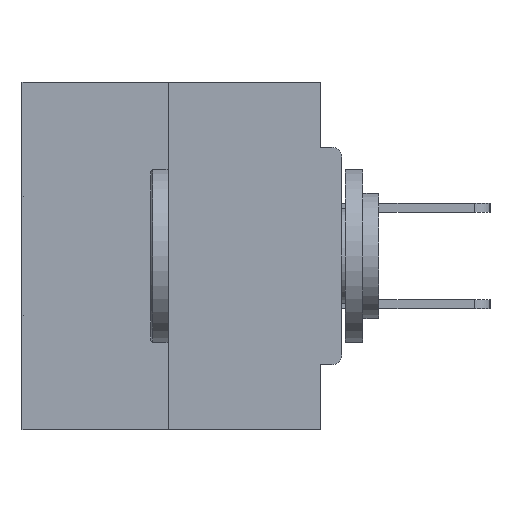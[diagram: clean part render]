
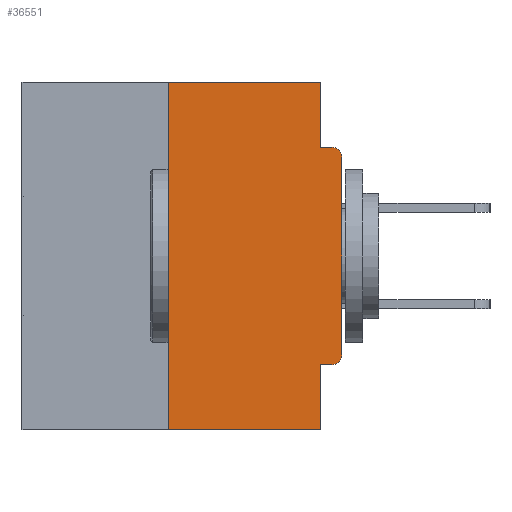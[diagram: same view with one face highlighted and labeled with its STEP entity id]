
A CAD part, left-side view. The second image highlights one B-rep face of the part: STEP entity #36551.
In plain terms, the highlighted planar face has unit normal (-1, 0, 0).
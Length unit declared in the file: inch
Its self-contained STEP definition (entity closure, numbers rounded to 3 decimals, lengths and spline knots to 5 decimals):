
#338 = DIRECTION ( 'NONE',  ( 0., -1., 0. ) ) ;
#385 = VECTOR ( 'NONE', #25717, 39.37008 ) ;
#518 = CARTESIAN_POINT ( 'NONE',  ( 0., 0.46, 0. ) ) ;
#1648 = DIRECTION ( 'NONE',  ( 0., 0., 1. ) ) ;
#1758 = CARTESIAN_POINT ( 'NONE',  ( 0., 0., 0. ) ) ;
#1766 = AXIS2_PLACEMENT_3D ( 'NONE', #30039, #36216, #30303 ) ;
#2018 = LINE ( 'NONE', #14596, #20647 ) ;
#2046 = CARTESIAN_POINT ( 'NONE',  ( 0., 0.25, -0.5 ) ) ;
#3592 = EDGE_CURVE ( 'NONE', #36708, #32702, #34409, .T. ) ;
#4123 = ORIENTED_EDGE ( 'NONE', *, *, #37410, .F. ) ;
#4656 = VECTOR ( 'NONE', #34241, 39.37008 ) ;
#4747 = CIRCLE ( 'NONE', #18517, 0.015 ) ;
#5923 = VERTEX_POINT ( 'NONE', #27540 ) ;
#6264 = CARTESIAN_POINT ( 'NONE',  ( 0., 0., -0.0935 ) ) ;
#6756 = VECTOR ( 'NONE', #338, 39.37008 ) ;
#6948 = ORIENTED_EDGE ( 'NONE', *, *, #17255, .F. ) ;
#7459 = DIRECTION ( 'NONE',  ( 1., 0., 0. ) ) ;
#8362 = EDGE_CURVE ( 'NONE', #36708, #20946, #20448, .T. ) ;
#8731 = CARTESIAN_POINT ( 'NONE',  ( 0., 0., -0.4065 ) ) ;
#9077 = LINE ( 'NONE', #6264, #6756 ) ;
#9250 = VERTEX_POINT ( 'NONE', #34932 ) ;
#9706 = ORIENTED_EDGE ( 'NONE', *, *, #15692, .T. ) ;
#9773 = VERTEX_POINT ( 'NONE', #11097 ) ;
#10700 = CARTESIAN_POINT ( 'NONE',  ( 0., 0.46, 0. ) ) ;
#11097 = CARTESIAN_POINT ( 'NONE',  ( 0., 0.015, -0.0935 ) ) ;
#11478 = LINE ( 'NONE', #518, #29188 ) ;
#11847 = CARTESIAN_POINT ( 'NONE',  ( 0., 0.031, -0.5 ) ) ;
#11968 = VECTOR ( 'NONE', #1648, 39.37008 ) ;
#11971 = CARTESIAN_POINT ( 'NONE',  ( 0., 0.015, -0.3915 ) ) ;
#12095 = DIRECTION ( 'NONE',  ( -1., 0., 0. ) ) ;
#14596 = CARTESIAN_POINT ( 'NONE',  ( 0., 0.031, 0. ) ) ;
#15692 = EDGE_CURVE ( 'NONE', #20719, #9773, #34105, .T. ) ;
#16983 = CARTESIAN_POINT ( 'NONE',  ( 0., 0.25, 0. ) ) ;
#17255 = EDGE_CURVE ( 'NONE', #5923, #20946, #37753, .T. ) ;
#17646 = CARTESIAN_POINT ( 'NONE',  ( 0., 0.015, -0.4065 ) ) ;
#18517 = AXIS2_PLACEMENT_3D ( 'NONE', #11971, #12095, #35986 ) ;
#19085 = ORIENTED_EDGE ( 'NONE', *, *, #19563, .F. ) ;
#19365 = PLANE ( 'NONE',  #24230 ) ;
#19563 = EDGE_CURVE ( 'NONE', #9250, #9773, #9077, .T. ) ;
#19780 = ORIENTED_EDGE ( 'NONE', *, *, #8362, .T. ) ;
#19796 = EDGE_CURVE ( 'NONE', #27564, #20719, #30009, .T. ) ;
#20267 = EDGE_LOOP ( 'NONE', ( #32837, #20473, #19780, #6948, #32783, #22545, #23385, #9706, #19085, #4123 ) ) ;
#20448 = LINE ( 'NONE', #31205, #4656 ) ;
#20473 = ORIENTED_EDGE ( 'NONE', *, *, #3592, .F. ) ;
#20647 = VECTOR ( 'NONE', #20677, 39.37008 ) ;
#20677 = DIRECTION ( 'NONE',  ( 0., 0., -1. ) ) ;
#20719 = VERTEX_POINT ( 'NONE', #34102 ) ;
#20946 = VERTEX_POINT ( 'NONE', #11847 ) ;
#20996 = EDGE_CURVE ( 'NONE', #27546, #5923, #31679, .T. ) ;
#21821 = VECTOR ( 'NONE', #32972, 39.37008 ) ;
#22545 = ORIENTED_EDGE ( 'NONE', *, *, #34361, .T. ) ;
#23385 = ORIENTED_EDGE ( 'NONE', *, *, #19796, .T. ) ;
#24230 = AXIS2_PLACEMENT_3D ( 'NONE', #10700, #7459, #31681 ) ;
#24546 = VERTEX_POINT ( 'NONE', #31802 ) ;
#25610 = DIRECTION ( 'NONE',  ( 0., 0., 1. ) ) ;
#25717 = DIRECTION ( 'NONE',  ( 0., 0., -1. ) ) ;
#25827 = FACE_OUTER_BOUND ( 'NONE', #20267, .T. ) ;
#26524 = CARTESIAN_POINT ( 'NONE',  ( 0., 0., -0.3915 ) ) ;
#27540 = CARTESIAN_POINT ( 'NONE',  ( 0., 0.031, -0.4065 ) ) ;
#27546 = VERTEX_POINT ( 'NONE', #17646 ) ;
#27564 = VERTEX_POINT ( 'NONE', #26524 ) ;
#28493 = CARTESIAN_POINT ( 'NONE',  ( 0., 0.031, -0.5 ) ) ;
#29188 = VECTOR ( 'NONE', #33545, 39.37008 ) ;
#30009 = LINE ( 'NONE', #1758, #32344 ) ;
#30039 = CARTESIAN_POINT ( 'NONE',  ( 0., 0.015, -0.1085 ) ) ;
#30303 = DIRECTION ( 'NONE',  ( 0., 0., -1. ) ) ;
#31205 = CARTESIAN_POINT ( 'NONE',  ( 0., 0.46, -0.5 ) ) ;
#31679 = LINE ( 'NONE', #8731, #21821 ) ;
#31681 = DIRECTION ( 'NONE',  ( 0., 0., -1. ) ) ;
#31802 = CARTESIAN_POINT ( 'NONE',  ( 0., 0.031, 0. ) ) ;
#32344 = VECTOR ( 'NONE', #25610, 39.37008 ) ;
#32702 = VERTEX_POINT ( 'NONE', #16983 ) ;
#32783 = ORIENTED_EDGE ( 'NONE', *, *, #20996, .F. ) ;
#32837 = ORIENTED_EDGE ( 'NONE', *, *, #35759, .F. ) ;
#32972 = DIRECTION ( 'NONE',  ( 0., 1., 0. ) ) ;
#33545 = DIRECTION ( 'NONE',  ( 0., -1., 0. ) ) ;
#34102 = CARTESIAN_POINT ( 'NONE',  ( 0., 0., -0.1085 ) ) ;
#34105 = CIRCLE ( 'NONE', #1766, 0.015 ) ;
#34241 = DIRECTION ( 'NONE',  ( 0., -1., 0. ) ) ;
#34361 = EDGE_CURVE ( 'NONE', #27546, #27564, #4747, .T. ) ;
#34409 = LINE ( 'NONE', #34430, #11968 ) ;
#34430 = CARTESIAN_POINT ( 'NONE',  ( 0., 0.25, 0. ) ) ;
#34932 = CARTESIAN_POINT ( 'NONE',  ( 0., 0.031, -0.0935 ) ) ;
#35759 = EDGE_CURVE ( 'NONE', #32702, #24546, #11478, .T. ) ;
#35986 = DIRECTION ( 'NONE',  ( 0., 0., -1. ) ) ;
#36216 = DIRECTION ( 'NONE',  ( -1., 0., 0. ) ) ;
#36551 = ADVANCED_FACE ( 'NONE', ( #25827 ), #19365, .F. ) ;
#36708 = VERTEX_POINT ( 'NONE', #2046 ) ;
#37410 = EDGE_CURVE ( 'NONE', #24546, #9250, #2018, .T. ) ;
#37753 = LINE ( 'NONE', #28493, #385 ) ;
